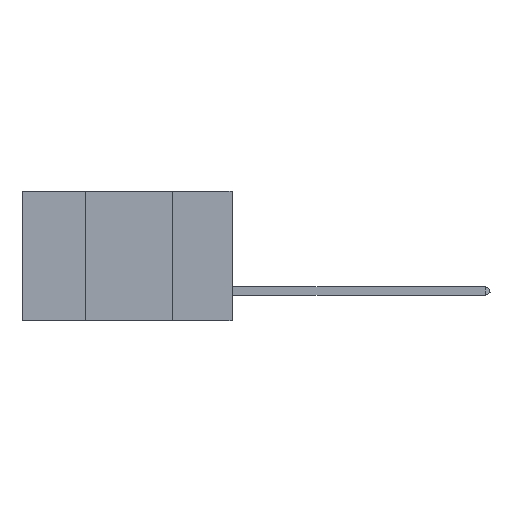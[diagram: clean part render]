
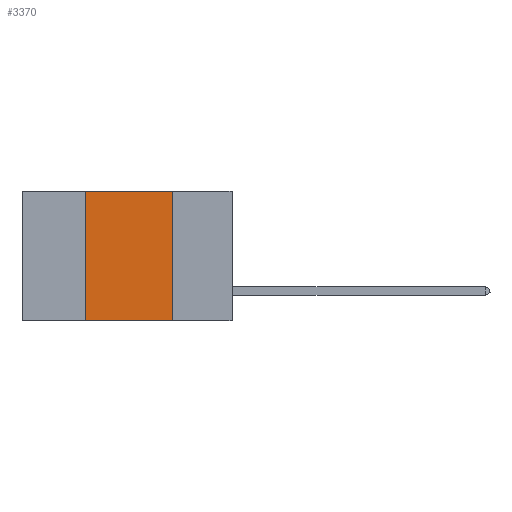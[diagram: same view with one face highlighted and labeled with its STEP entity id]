
A CAD part, left-side view. The second image highlights one B-rep face of the part: STEP entity #3370.
In plain terms, the highlighted planar face has unit normal (-1, 0, 0).
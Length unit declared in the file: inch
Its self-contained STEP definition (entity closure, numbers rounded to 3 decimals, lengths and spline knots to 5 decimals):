
#111 = VECTOR ( 'NONE', #13785, 39.37008 ) ;
#371 = ORIENTED_EDGE ( 'NONE', *, *, #9083, .F. ) ;
#1025 = DIRECTION ( 'NONE',  ( 0., -1., 0. ) ) ;
#1299 = CARTESIAN_POINT ( 'NONE',  ( 0., 0.17, 0. ) ) ;
#2131 = LINE ( 'NONE', #4491, #13937 ) ;
#2229 = DIRECTION ( 'NONE',  ( 1., 0., 0. ) ) ;
#2915 = LINE ( 'NONE', #1299, #111 ) ;
#2973 = VERTEX_POINT ( 'NONE', #11965 ) ;
#3185 = CARTESIAN_POINT ( 'NONE',  ( 0., 0.42, 0. ) ) ;
#3308 = CARTESIAN_POINT ( 'NONE',  ( 0., 0.42, 0. ) ) ;
#3370 = ADVANCED_FACE ( 'NONE', ( #7687 ), #6992, .F. ) ;
#3398 = DIRECTION ( 'NONE',  ( 0., -1., 0. ) ) ;
#3401 = VECTOR ( 'NONE', #1025, 39.37008 ) ;
#4146 = ORIENTED_EDGE ( 'NONE', *, *, #15705, .F. ) ;
#4432 = DIRECTION ( 'NONE',  ( 0., 0., 1. ) ) ;
#4491 = CARTESIAN_POINT ( 'NONE',  ( 0., 0.6, -0.37 ) ) ;
#6361 = CARTESIAN_POINT ( 'NONE',  ( 0., 0.42, -0.37 ) ) ;
#6727 = LINE ( 'NONE', #7441, #3401 ) ;
#6992 = PLANE ( 'NONE',  #14397 ) ;
#7032 = VECTOR ( 'NONE', #4432, 39.37008 ) ;
#7441 = CARTESIAN_POINT ( 'NONE',  ( 0., 0.6, 0. ) ) ;
#7687 = FACE_OUTER_BOUND ( 'NONE', #9526, .T. ) ;
#9083 = EDGE_CURVE ( 'NONE', #16198, #2973, #6727, .T. ) ;
#9526 = EDGE_LOOP ( 'NONE', ( #12192, #371, #4146, #12382 ) ) ;
#9740 = CARTESIAN_POINT ( 'NONE',  ( 0., 0.6, 0. ) ) ;
#11396 = EDGE_CURVE ( 'NONE', #2973, #12395, #2915, .T. ) ;
#11965 = CARTESIAN_POINT ( 'NONE',  ( 0., 0.17, 0. ) ) ;
#12192 = ORIENTED_EDGE ( 'NONE', *, *, #11396, .F. ) ;
#12205 = DIRECTION ( 'NONE',  ( 0., 0., -1. ) ) ;
#12382 = ORIENTED_EDGE ( 'NONE', *, *, #15904, .T. ) ;
#12395 = VERTEX_POINT ( 'NONE', #14602 ) ;
#13555 = LINE ( 'NONE', #3308, #7032 ) ;
#13785 = DIRECTION ( 'NONE',  ( 0., 0., -1. ) ) ;
#13937 = VECTOR ( 'NONE', #3398, 39.37008 ) ;
#14397 = AXIS2_PLACEMENT_3D ( 'NONE', #9740, #2229, #12205 ) ;
#14489 = VERTEX_POINT ( 'NONE', #6361 ) ;
#14602 = CARTESIAN_POINT ( 'NONE',  ( 0., 0.17, -0.37 ) ) ;
#15705 = EDGE_CURVE ( 'NONE', #14489, #16198, #13555, .T. ) ;
#15904 = EDGE_CURVE ( 'NONE', #14489, #12395, #2131, .T. ) ;
#16198 = VERTEX_POINT ( 'NONE', #3185 ) ;
